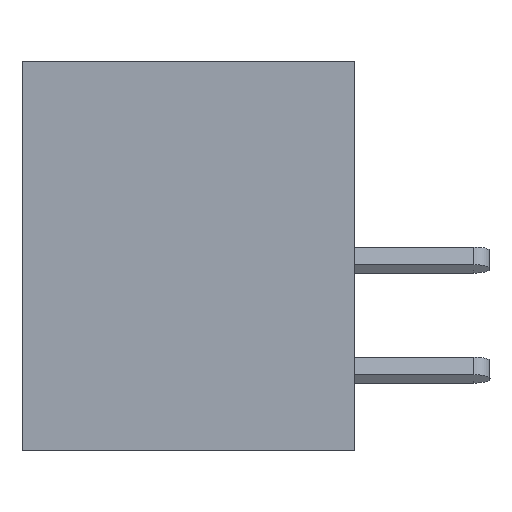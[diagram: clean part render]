
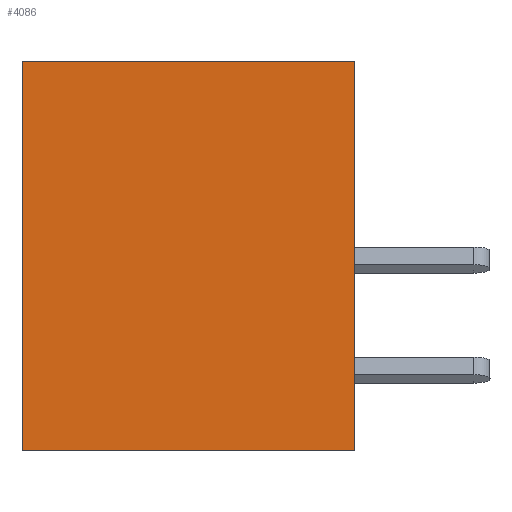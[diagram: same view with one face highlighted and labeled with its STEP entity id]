
A CAD part, left-side view. The second image highlights one B-rep face of the part: STEP entity #4086.
In plain terms, the highlighted planar face has unit normal (-1, 0, 0).
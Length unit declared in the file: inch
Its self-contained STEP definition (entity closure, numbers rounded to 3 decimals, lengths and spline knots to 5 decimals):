
#1262 = EDGE_CURVE ( 'NONE', #25421, #22124, #16479, .T. ) ;
#1522 = CARTESIAN_POINT ( 'NONE',  ( 0., 0., -0.531 ) ) ;
#1981 = VECTOR ( 'NONE', #18053, 39.37008 ) ;
#3007 = CARTESIAN_POINT ( 'NONE',  ( 0., 0., 0. ) ) ;
#3328 = LINE ( 'NONE', #3007, #1981 ) ;
#4086 = ADVANCED_FACE ( 'NONE', ( #17911 ), #27115, .F. ) ;
#4369 = VECTOR ( 'NONE', #15561, 39.37008 ) ;
#5018 = EDGE_CURVE ( 'NONE', #22372, #24288, #24936, .T. ) ;
#6541 = CARTESIAN_POINT ( 'NONE',  ( 0., 0.453, -0.531 ) ) ;
#6786 = CARTESIAN_POINT ( 'NONE',  ( 0., 0.453, 0. ) ) ;
#8379 = VECTOR ( 'NONE', #8813, 39.37008 ) ;
#8813 = DIRECTION ( 'NONE',  ( 0., -1., 0. ) ) ;
#9633 = ORIENTED_EDGE ( 'NONE', *, *, #5018, .F. ) ;
#11961 = CARTESIAN_POINT ( 'NONE',  ( 0., 0.453, 0. ) ) ;
#14421 = DIRECTION ( 'NONE',  ( 0., 0., -1. ) ) ;
#15345 = DIRECTION ( 'NONE',  ( 0., 0., 1. ) ) ;
#15561 = DIRECTION ( 'NONE',  ( 0., -1., 0. ) ) ;
#15568 = AXIS2_PLACEMENT_3D ( 'NONE', #11961, #22873, #14421 ) ;
#16479 = LINE ( 'NONE', #26352, #8379 ) ;
#17911 = FACE_OUTER_BOUND ( 'NONE', #19331, .T. ) ;
#18053 = DIRECTION ( 'NONE',  ( 0., 0., 1. ) ) ;
#18209 = ORIENTED_EDGE ( 'NONE', *, *, #27638, .F. ) ;
#19109 = CARTESIAN_POINT ( 'NONE',  ( 0., 0., 0. ) ) ;
#19331 = EDGE_LOOP ( 'NONE', ( #26815, #9633, #18209, #27677 ) ) ;
#22124 = VERTEX_POINT ( 'NONE', #1522 ) ;
#22372 = VERTEX_POINT ( 'NONE', #25223 ) ;
#22873 = DIRECTION ( 'NONE',  ( 1., 0., 0. ) ) ;
#23468 = CARTESIAN_POINT ( 'NONE',  ( 0., 0.453, 0. ) ) ;
#24288 = VERTEX_POINT ( 'NONE', #19109 ) ;
#24936 = LINE ( 'NONE', #23468, #4369 ) ;
#25223 = CARTESIAN_POINT ( 'NONE',  ( 0., 0.453, 0. ) ) ;
#25421 = VERTEX_POINT ( 'NONE', #6541 ) ;
#25539 = LINE ( 'NONE', #6786, #26877 ) ;
#26352 = CARTESIAN_POINT ( 'NONE',  ( 0., 0.453, -0.531 ) ) ;
#26630 = EDGE_CURVE ( 'NONE', #22124, #24288, #3328, .T. ) ;
#26815 = ORIENTED_EDGE ( 'NONE', *, *, #26630, .T. ) ;
#26877 = VECTOR ( 'NONE', #15345, 39.37008 ) ;
#27115 = PLANE ( 'NONE',  #15568 ) ;
#27638 = EDGE_CURVE ( 'NONE', #25421, #22372, #25539, .T. ) ;
#27677 = ORIENTED_EDGE ( 'NONE', *, *, #1262, .T. ) ;
